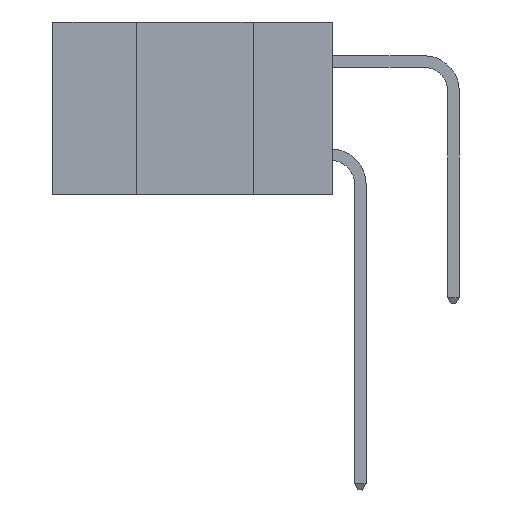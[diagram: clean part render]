
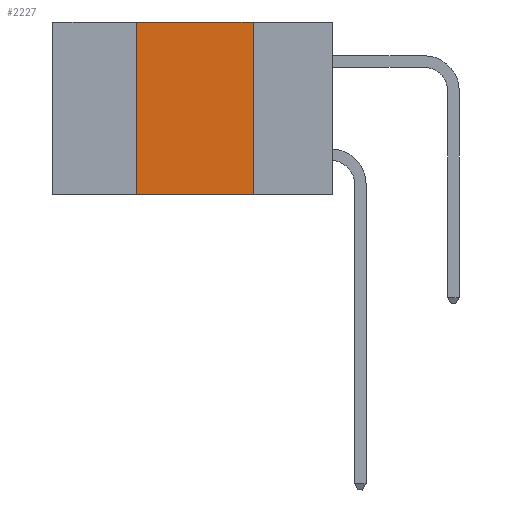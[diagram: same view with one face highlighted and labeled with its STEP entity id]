
A CAD part, left-side view. The second image highlights one B-rep face of the part: STEP entity #2227.
In plain terms, the highlighted planar face has unit normal (-1, 0, 0).
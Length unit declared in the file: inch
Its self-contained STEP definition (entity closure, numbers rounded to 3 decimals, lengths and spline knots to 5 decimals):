
#1247 = DIRECTION ( 'NONE',  ( 1., 0., 0. ) ) ;
#1480 = DIRECTION ( 'NONE',  ( 0., 0., -1. ) ) ;
#1642 = LINE ( 'NONE', #9690, #16403 ) ;
#1774 = DIRECTION ( 'NONE',  ( 0., 0., -1. ) ) ;
#2227 = ADVANCED_FACE ( 'NONE', ( #3049 ), #12492, .F. ) ;
#3049 = FACE_OUTER_BOUND ( 'NONE', #14848, .T. ) ;
#3175 = LINE ( 'NONE', #14085, #17819 ) ;
#3352 = VECTOR ( 'NONE', #1480, 39.37008 ) ;
#3755 = DIRECTION ( 'NONE',  ( 0., -1., 0. ) ) ;
#4456 = CARTESIAN_POINT ( 'NONE',  ( 0., 0.17, 0. ) ) ;
#4839 = VERTEX_POINT ( 'NONE', #4456 ) ;
#4936 = ORIENTED_EDGE ( 'NONE', *, *, #13843, .F. ) ;
#7106 = ORIENTED_EDGE ( 'NONE', *, *, #14172, .T. ) ;
#7427 = CARTESIAN_POINT ( 'NONE',  ( 0., 0.17, 0. ) ) ;
#8449 = AXIS2_PLACEMENT_3D ( 'NONE', #17390, #1247, #1774 ) ;
#8970 = ORIENTED_EDGE ( 'NONE', *, *, #15750, .F. ) ;
#9690 = CARTESIAN_POINT ( 'NONE',  ( 0., 0.6, -0.37 ) ) ;
#11814 = CARTESIAN_POINT ( 'NONE',  ( 0., 0.42, -0.37 ) ) ;
#11995 = CARTESIAN_POINT ( 'NONE',  ( 0., 0.42, 0. ) ) ;
#12310 = EDGE_CURVE ( 'NONE', #17764, #4839, #3175, .T. ) ;
#12492 = PLANE ( 'NONE',  #8449 ) ;
#13141 = ORIENTED_EDGE ( 'NONE', *, *, #12310, .F. ) ;
#13520 = DIRECTION ( 'NONE',  ( 0., 0., 1. ) ) ;
#13808 = VERTEX_POINT ( 'NONE', #11814 ) ;
#13843 = EDGE_CURVE ( 'NONE', #4839, #15124, #15076, .T. ) ;
#14085 = CARTESIAN_POINT ( 'NONE',  ( 0., 0.6, 0. ) ) ;
#14172 = EDGE_CURVE ( 'NONE', #13808, #15124, #1642, .T. ) ;
#14848 = EDGE_LOOP ( 'NONE', ( #4936, #13141, #8970, #7106 ) ) ;
#15029 = CARTESIAN_POINT ( 'NONE',  ( 0., 0.17, -0.37 ) ) ;
#15076 = LINE ( 'NONE', #7427, #3352 ) ;
#15124 = VERTEX_POINT ( 'NONE', #15029 ) ;
#15439 = VECTOR ( 'NONE', #13520, 39.37008 ) ;
#15750 = EDGE_CURVE ( 'NONE', #13808, #17764, #18345, .T. ) ;
#16403 = VECTOR ( 'NONE', #16986, 39.37008 ) ;
#16986 = DIRECTION ( 'NONE',  ( 0., -1., 0. ) ) ;
#17390 = CARTESIAN_POINT ( 'NONE',  ( 0., 0.6, 0. ) ) ;
#17764 = VERTEX_POINT ( 'NONE', #18484 ) ;
#17819 = VECTOR ( 'NONE', #3755, 39.37008 ) ;
#18345 = LINE ( 'NONE', #11995, #15439 ) ;
#18484 = CARTESIAN_POINT ( 'NONE',  ( 0., 0.42, 0. ) ) ;
